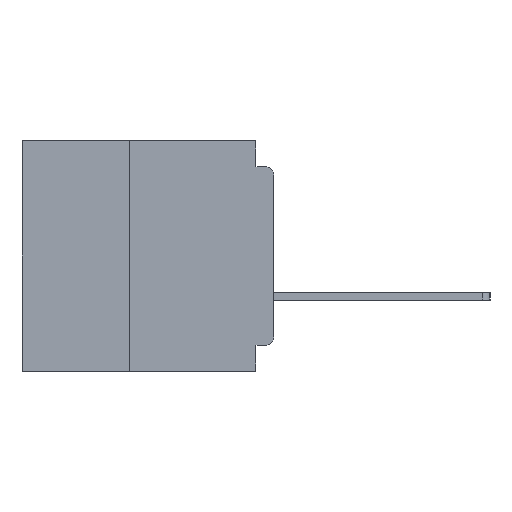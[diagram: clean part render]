
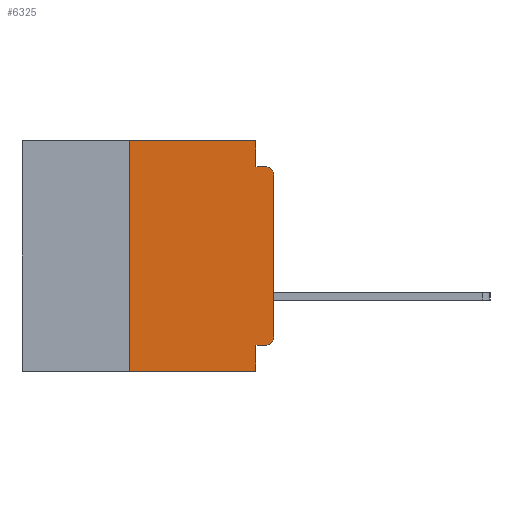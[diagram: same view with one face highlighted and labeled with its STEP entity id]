
A CAD part, left-side view. The second image highlights one B-rep face of the part: STEP entity #6325.
In plain terms, the highlighted planar face has unit normal (-1, 0, 0).
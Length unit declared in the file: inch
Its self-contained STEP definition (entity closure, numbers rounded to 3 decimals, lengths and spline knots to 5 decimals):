
#369 = LINE ( 'NONE', #9055, #7844 ) ;
#370 = EDGE_LOOP ( 'NONE', ( #40973, #1965, #3895, #11958, #8277, #5516, #39571, #38404, #12147, #7965 ) ) ;
#1965 = ORIENTED_EDGE ( 'NONE', *, *, #4529, .T. ) ;
#2169 = CARTESIAN_POINT ( 'NONE',  ( 0., 0.25, -0.4 ) ) ;
#2484 = DIRECTION ( 'NONE',  ( 0., 0., -1. ) ) ;
#3895 = ORIENTED_EDGE ( 'NONE', *, *, #36645, .F. ) ;
#4470 = LINE ( 'NONE', #12787, #35499 ) ;
#4529 = EDGE_CURVE ( 'NONE', #40600, #4773, #11333, .T. ) ;
#4773 = VERTEX_POINT ( 'NONE', #5924 ) ;
#4776 = CARTESIAN_POINT ( 'NONE',  ( 0., 0.031, 0. ) ) ;
#4972 = DIRECTION ( 'NONE',  ( 0., 0., -1. ) ) ;
#5398 = DIRECTION ( 'NONE',  ( 0., 0., 1. ) ) ;
#5516 = ORIENTED_EDGE ( 'NONE', *, *, #35800, .F. ) ;
#5827 = VECTOR ( 'NONE', #15384, 39.37008 ) ;
#5924 = CARTESIAN_POINT ( 'NONE',  ( 0., 0.015, -0.045 ) ) ;
#6325 = ADVANCED_FACE ( 'NONE', ( #17682 ), #20997, .F. ) ;
#6337 = DIRECTION ( 'NONE',  ( 0., -1., 0. ) ) ;
#6510 = CARTESIAN_POINT ( 'NONE',  ( 0., 0.031, -0.355 ) ) ;
#6600 = EDGE_CURVE ( 'NONE', #25562, #33369, #9245, .T. ) ;
#7844 = VECTOR ( 'NONE', #34652, 39.37008 ) ;
#7965 = ORIENTED_EDGE ( 'NONE', *, *, #39483, .T. ) ;
#7990 = DIRECTION ( 'NONE',  ( 0., 0., -1. ) ) ;
#8277 = ORIENTED_EDGE ( 'NONE', *, *, #6600, .F. ) ;
#9055 = CARTESIAN_POINT ( 'NONE',  ( 0., 0., -0.355 ) ) ;
#9245 = LINE ( 'NONE', #35027, #34777 ) ;
#9303 = AXIS2_PLACEMENT_3D ( 'NONE', #23924, #24209, #4972 ) ;
#10181 = EDGE_CURVE ( 'NONE', #14803, #40600, #4470, .T. ) ;
#10617 = CARTESIAN_POINT ( 'NONE',  ( 0., 0.031, 0. ) ) ;
#11244 = VECTOR ( 'NONE', #7990, 39.37008 ) ;
#11333 = CIRCLE ( 'NONE', #37797, 0.015 ) ;
#11958 = ORIENTED_EDGE ( 'NONE', *, *, #39941, .F. ) ;
#12147 = ORIENTED_EDGE ( 'NONE', *, *, #17446, .F. ) ;
#12787 = CARTESIAN_POINT ( 'NONE',  ( 0., 0., 0. ) ) ;
#14671 = CARTESIAN_POINT ( 'NONE',  ( 0., 0., -0.34 ) ) ;
#14803 = VERTEX_POINT ( 'NONE', #14671 ) ;
#15384 = DIRECTION ( 'NONE',  ( 0., -1., 0. ) ) ;
#16039 = DIRECTION ( 'NONE',  ( 0., 0., 1. ) ) ;
#17446 = EDGE_CURVE ( 'NONE', #38951, #21381, #369, .T. ) ;
#17654 = LINE ( 'NONE', #40614, #33636 ) ;
#17682 = FACE_OUTER_BOUND ( 'NONE', #370, .T. ) ;
#17740 = DIRECTION ( 'NONE',  ( -1., 0., 0. ) ) ;
#17936 = CARTESIAN_POINT ( 'NONE',  ( 0., 0., -0.06 ) ) ;
#18599 = CARTESIAN_POINT ( 'NONE',  ( 0., 0.015, -0.34 ) ) ;
#19037 = CARTESIAN_POINT ( 'NONE',  ( 0., 0.031, -0.4 ) ) ;
#19284 = AXIS2_PLACEMENT_3D ( 'NONE', #18599, #40699, #21817 ) ;
#19438 = CARTESIAN_POINT ( 'NONE',  ( 0., 0.25, 0. ) ) ;
#20997 = PLANE ( 'NONE',  #9303 ) ;
#21327 = VERTEX_POINT ( 'NONE', #19037 ) ;
#21381 = VERTEX_POINT ( 'NONE', #6510 ) ;
#21817 = DIRECTION ( 'NONE',  ( 0., 0., -1. ) ) ;
#22257 = VERTEX_POINT ( 'NONE', #36725 ) ;
#22728 = VECTOR ( 'NONE', #5398, 39.37008 ) ;
#23924 = CARTESIAN_POINT ( 'NONE',  ( 0., 0.437, 0. ) ) ;
#24209 = DIRECTION ( 'NONE',  ( 1., 0., 0. ) ) ;
#25017 = LINE ( 'NONE', #32072, #40767 ) ;
#25562 = VERTEX_POINT ( 'NONE', #19438 ) ;
#27272 = EDGE_CURVE ( 'NONE', #21381, #21327, #17654, .T. ) ;
#28233 = LINE ( 'NONE', #4776, #11244 ) ;
#31142 = CARTESIAN_POINT ( 'NONE',  ( 0., 0.25, -0.4 ) ) ;
#32072 = CARTESIAN_POINT ( 'NONE',  ( 0., 0., -0.045 ) ) ;
#32181 = LINE ( 'NONE', #2169, #22728 ) ;
#33369 = VERTEX_POINT ( 'NONE', #10617 ) ;
#33636 = VECTOR ( 'NONE', #2484, 39.37008 ) ;
#33698 = EDGE_CURVE ( 'NONE', #39024, #21327, #39692, .T. ) ;
#34652 = DIRECTION ( 'NONE',  ( 0., 1., 0. ) ) ;
#34777 = VECTOR ( 'NONE', #6337, 39.37008 ) ;
#34817 = CARTESIAN_POINT ( 'NONE',  ( 0., 0.015, -0.355 ) ) ;
#35027 = CARTESIAN_POINT ( 'NONE',  ( 0., 0.437, 0. ) ) ;
#35275 = DIRECTION ( 'NONE',  ( 0., -1., 0. ) ) ;
#35499 = VECTOR ( 'NONE', #16039, 39.37008 ) ;
#35736 = CIRCLE ( 'NONE', #19284, 0.015 ) ;
#35800 = EDGE_CURVE ( 'NONE', #39024, #25562, #32181, .T. ) ;
#36645 = EDGE_CURVE ( 'NONE', #22257, #4773, #25017, .T. ) ;
#36725 = CARTESIAN_POINT ( 'NONE',  ( 0., 0.031, -0.045 ) ) ;
#36787 = CARTESIAN_POINT ( 'NONE',  ( 0., 0.015, -0.06 ) ) ;
#37603 = CARTESIAN_POINT ( 'NONE',  ( 0., 0.437, -0.4 ) ) ;
#37797 = AXIS2_PLACEMENT_3D ( 'NONE', #36787, #17740, #39900 ) ;
#38404 = ORIENTED_EDGE ( 'NONE', *, *, #27272, .F. ) ;
#38951 = VERTEX_POINT ( 'NONE', #34817 ) ;
#39024 = VERTEX_POINT ( 'NONE', #31142 ) ;
#39483 = EDGE_CURVE ( 'NONE', #38951, #14803, #35736, .T. ) ;
#39571 = ORIENTED_EDGE ( 'NONE', *, *, #33698, .T. ) ;
#39692 = LINE ( 'NONE', #37603, #5827 ) ;
#39900 = DIRECTION ( 'NONE',  ( 0., 0., -1. ) ) ;
#39941 = EDGE_CURVE ( 'NONE', #33369, #22257, #28233, .T. ) ;
#40600 = VERTEX_POINT ( 'NONE', #17936 ) ;
#40614 = CARTESIAN_POINT ( 'NONE',  ( 0., 0.031, -0.4 ) ) ;
#40699 = DIRECTION ( 'NONE',  ( -1., 0., 0. ) ) ;
#40767 = VECTOR ( 'NONE', #35275, 39.37008 ) ;
#40973 = ORIENTED_EDGE ( 'NONE', *, *, #10181, .T. ) ;
